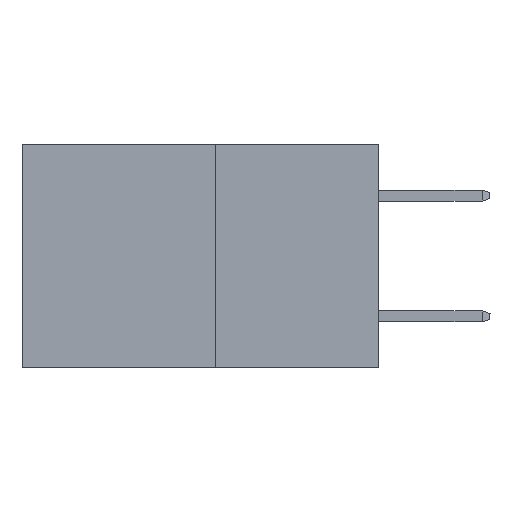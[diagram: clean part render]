
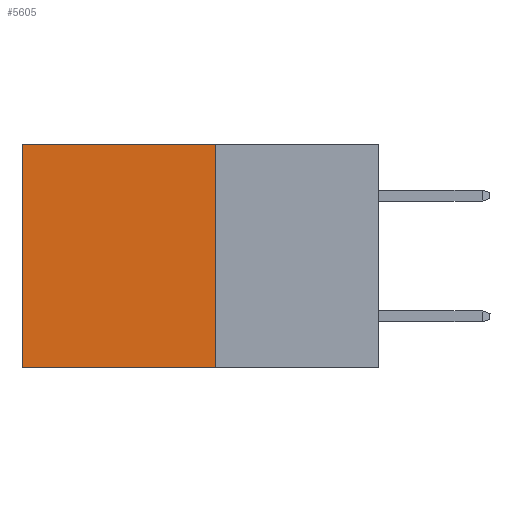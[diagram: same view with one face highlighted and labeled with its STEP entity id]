
A CAD part, left-side view. The second image highlights one B-rep face of the part: STEP entity #5605.
In plain terms, the highlighted planar face has unit normal (-1, 0, 0).
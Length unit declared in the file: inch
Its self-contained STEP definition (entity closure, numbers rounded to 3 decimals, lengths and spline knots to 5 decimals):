
#266 = EDGE_CURVE ( 'NONE', #4114, #5757, #8596, .T. ) ;
#804 = CARTESIAN_POINT ( 'NONE',  ( 0.277, 0.27, -0.37 ) ) ;
#1010 = ORIENTED_EDGE ( 'NONE', *, *, #266, .F. ) ;
#1724 = LINE ( 'NONE', #12939, #15558 ) ;
#2595 = CARTESIAN_POINT ( 'NONE',  ( 0.277, 0.59, 0. ) ) ;
#2636 = CARTESIAN_POINT ( 'NONE',  ( 0.277, 0.59, -0.37 ) ) ;
#2694 = VECTOR ( 'NONE', #6938, 39.37008 ) ;
#3206 = EDGE_CURVE ( 'NONE', #5757, #4303, #1724, .T. ) ;
#4114 = VERTEX_POINT ( 'NONE', #7061 ) ;
#4303 = VERTEX_POINT ( 'NONE', #10741 ) ;
#5000 = VECTOR ( 'NONE', #5085, 39.37008 ) ;
#5085 = DIRECTION ( 'NONE',  ( 0., 0., -1. ) ) ;
#5149 = EDGE_CURVE ( 'NONE', #4114, #11749, #6231, .T. ) ;
#5605 = ADVANCED_FACE ( 'NONE', ( #5794 ), #15945, .F. ) ;
#5757 = VERTEX_POINT ( 'NONE', #14256 ) ;
#5794 = FACE_OUTER_BOUND ( 'NONE', #9312, .T. ) ;
#5912 = LINE ( 'NONE', #2636, #15794 ) ;
#6231 = LINE ( 'NONE', #6787, #2694 ) ;
#6765 = CARTESIAN_POINT ( 'NONE',  ( 0.277, 0.27, -0.37 ) ) ;
#6787 = CARTESIAN_POINT ( 'NONE',  ( 0.277, 0.27, 0. ) ) ;
#6938 = DIRECTION ( 'NONE',  ( 0., 1., 0. ) ) ;
#7061 = CARTESIAN_POINT ( 'NONE',  ( 0.277, 0.27, 0. ) ) ;
#8596 = LINE ( 'NONE', #6765, #5000 ) ;
#9312 = EDGE_LOOP ( 'NONE', ( #13970, #14405, #1010, #11664 ) ) ;
#10452 = DIRECTION ( 'NONE',  ( 0., 1., 0. ) ) ;
#10741 = CARTESIAN_POINT ( 'NONE',  ( 0.277, 0.59, -0.37 ) ) ;
#11664 = ORIENTED_EDGE ( 'NONE', *, *, #5149, .T. ) ;
#11749 = VERTEX_POINT ( 'NONE', #2595 ) ;
#12323 = EDGE_CURVE ( 'NONE', #11749, #4303, #5912, .T. ) ;
#12939 = CARTESIAN_POINT ( 'NONE',  ( 0.277, 0.27, -0.37 ) ) ;
#13277 = DIRECTION ( 'NONE',  ( 0., 0., -1. ) ) ;
#13970 = ORIENTED_EDGE ( 'NONE', *, *, #12323, .T. ) ;
#14031 = AXIS2_PLACEMENT_3D ( 'NONE', #804, #15625, #15602 ) ;
#14256 = CARTESIAN_POINT ( 'NONE',  ( 0.277, 0.27, -0.37 ) ) ;
#14405 = ORIENTED_EDGE ( 'NONE', *, *, #3206, .F. ) ;
#15558 = VECTOR ( 'NONE', #10452, 39.37008 ) ;
#15602 = DIRECTION ( 'NONE',  ( 0., 0., -1. ) ) ;
#15625 = DIRECTION ( 'NONE',  ( 1., 0., 0. ) ) ;
#15794 = VECTOR ( 'NONE', #13277, 39.37008 ) ;
#15945 = PLANE ( 'NONE',  #14031 ) ;
